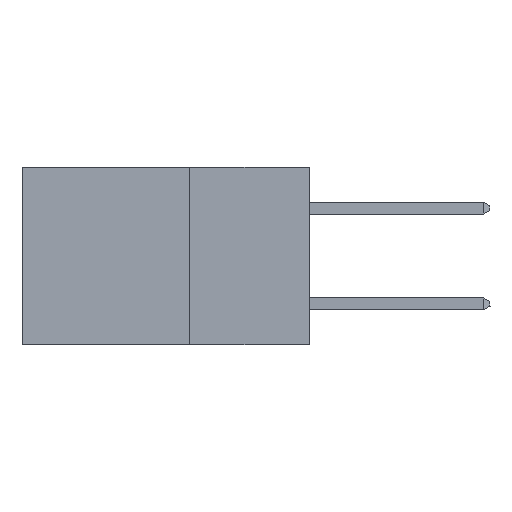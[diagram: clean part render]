
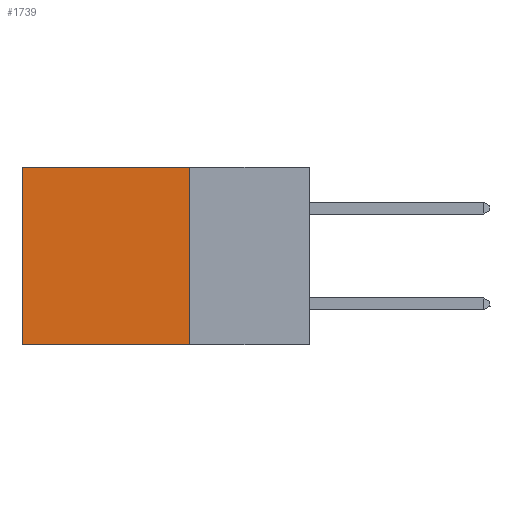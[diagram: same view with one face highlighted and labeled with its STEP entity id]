
A CAD part, left-side view. The second image highlights one B-rep face of the part: STEP entity #1739.
In plain terms, the highlighted planar face has unit normal (-1, 0, 0).
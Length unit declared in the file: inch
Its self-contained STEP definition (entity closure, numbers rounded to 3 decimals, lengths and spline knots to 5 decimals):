
#236 = CARTESIAN_POINT ( 'NONE',  ( 0.2875, 0.6, 0. ) ) ;
#263 = CARTESIAN_POINT ( 'NONE',  ( 0.2875, 0.6, 0. ) ) ;
#580 = FACE_OUTER_BOUND ( 'NONE', #10264, .T. ) ;
#948 = DIRECTION ( 'NONE',  ( 0., 1., 0. ) ) ;
#1026 = DIRECTION ( 'NONE',  ( 0., 0., -1. ) ) ;
#1517 = VECTOR ( 'NONE', #948, 39.37008 ) ;
#1596 = LINE ( 'NONE', #13150, #9429 ) ;
#1739 = ADVANCED_FACE ( 'NONE', ( #580 ), #6650, .F. ) ;
#1837 = DIRECTION ( 'NONE',  ( 0., 1., 0. ) ) ;
#1915 = EDGE_CURVE ( 'NONE', #5305, #14511, #13248, .T. ) ;
#2092 = CARTESIAN_POINT ( 'NONE',  ( 0.2875, 0.25, 0. ) ) ;
#3219 = CARTESIAN_POINT ( 'NONE',  ( 0.2875, 0.25, -0.37 ) ) ;
#3669 = CARTESIAN_POINT ( 'NONE',  ( 0.2875, 0.6, -0.37 ) ) ;
#4887 = LINE ( 'NONE', #3219, #1517 ) ;
#5136 = EDGE_CURVE ( 'NONE', #6316, #5993, #11401, .T. ) ;
#5305 = VERTEX_POINT ( 'NONE', #263 ) ;
#5335 = ORIENTED_EDGE ( 'NONE', *, *, #7352, .F. ) ;
#5947 = CARTESIAN_POINT ( 'NONE',  ( 0.2875, 0.25, -0.37 ) ) ;
#5993 = VERTEX_POINT ( 'NONE', #5947 ) ;
#6217 = ORIENTED_EDGE ( 'NONE', *, *, #13304, .T. ) ;
#6316 = VERTEX_POINT ( 'NONE', #8140 ) ;
#6650 = PLANE ( 'NONE',  #10012 ) ;
#7352 = EDGE_CURVE ( 'NONE', #5993, #14511, #4887, .T. ) ;
#7534 = ORIENTED_EDGE ( 'NONE', *, *, #5136, .F. ) ;
#7976 = DIRECTION ( 'NONE',  ( 0., 0., -1. ) ) ;
#8140 = CARTESIAN_POINT ( 'NONE',  ( 0.2875, 0.25, 0. ) ) ;
#9429 = VECTOR ( 'NONE', #1837, 39.37008 ) ;
#9692 = DIRECTION ( 'NONE',  ( 0., 0., -1. ) ) ;
#9937 = ORIENTED_EDGE ( 'NONE', *, *, #1915, .T. ) ;
#10012 = AXIS2_PLACEMENT_3D ( 'NONE', #2092, #11239, #1026 ) ;
#10248 = VECTOR ( 'NONE', #9692, 39.37008 ) ;
#10264 = EDGE_LOOP ( 'NONE', ( #9937, #5335, #7534, #6217 ) ) ;
#11239 = DIRECTION ( 'NONE',  ( 1., 0., 0. ) ) ;
#11401 = LINE ( 'NONE', #13766, #14227 ) ;
#13150 = CARTESIAN_POINT ( 'NONE',  ( 0.2875, 0.25, 0. ) ) ;
#13248 = LINE ( 'NONE', #236, #10248 ) ;
#13304 = EDGE_CURVE ( 'NONE', #6316, #5305, #1596, .T. ) ;
#13766 = CARTESIAN_POINT ( 'NONE',  ( 0.2875, 0.25, 0. ) ) ;
#14227 = VECTOR ( 'NONE', #7976, 39.37008 ) ;
#14511 = VERTEX_POINT ( 'NONE', #3669 ) ;
